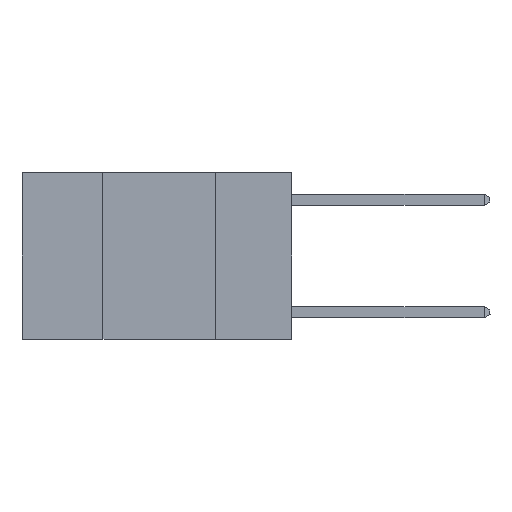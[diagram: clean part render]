
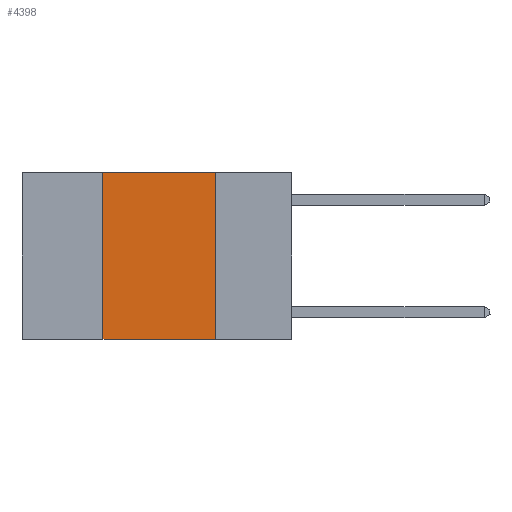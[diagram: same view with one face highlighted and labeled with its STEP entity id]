
A CAD part, left-side view. The second image highlights one B-rep face of the part: STEP entity #4398.
In plain terms, the highlighted planar face has unit normal (-1, 0, 0).
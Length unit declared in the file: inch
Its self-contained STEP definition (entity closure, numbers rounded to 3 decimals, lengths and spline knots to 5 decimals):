
#544 = CARTESIAN_POINT ( 'NONE',  ( 0., 0.17, 0. ) ) ;
#612 = CARTESIAN_POINT ( 'NONE',  ( 0., 0.17, -0.37 ) ) ;
#868 = EDGE_CURVE ( 'NONE', #10173, #6246, #11336, .T. ) ;
#2026 = VECTOR ( 'NONE', #4813, 39.37008 ) ;
#2029 = ORIENTED_EDGE ( 'NONE', *, *, #3747, .F. ) ;
#2306 = VERTEX_POINT ( 'NONE', #544 ) ;
#2623 = VECTOR ( 'NONE', #9434, 39.37008 ) ;
#3747 = EDGE_CURVE ( 'NONE', #2306, #5286, #10767, .T. ) ;
#3862 = EDGE_CURVE ( 'NONE', #10173, #5286, #4146, .T. ) ;
#3988 = ORIENTED_EDGE ( 'NONE', *, *, #3862, .T. ) ;
#4146 = LINE ( 'NONE', #8039, #8709 ) ;
#4253 = CARTESIAN_POINT ( 'NONE',  ( 0., 0.42, 0. ) ) ;
#4398 = ADVANCED_FACE ( 'NONE', ( #5860 ), #8008, .F. ) ;
#4813 = DIRECTION ( 'NONE',  ( 0., 0., 1. ) ) ;
#5286 = VERTEX_POINT ( 'NONE', #612 ) ;
#5776 = EDGE_CURVE ( 'NONE', #6246, #2306, #7367, .T. ) ;
#5856 = VECTOR ( 'NONE', #11482, 39.37008 ) ;
#5860 = FACE_OUTER_BOUND ( 'NONE', #10255, .T. ) ;
#6067 = CARTESIAN_POINT ( 'NONE',  ( 0., 0.42, -0.37 ) ) ;
#6246 = VERTEX_POINT ( 'NONE', #7239 ) ;
#7239 = CARTESIAN_POINT ( 'NONE',  ( 0., 0.42, 0. ) ) ;
#7367 = LINE ( 'NONE', #7677, #2623 ) ;
#7477 = AXIS2_PLACEMENT_3D ( 'NONE', #7942, #7882, #7865 ) ;
#7677 = CARTESIAN_POINT ( 'NONE',  ( 0., 0.6, 0. ) ) ;
#7780 = ORIENTED_EDGE ( 'NONE', *, *, #868, .F. ) ;
#7865 = DIRECTION ( 'NONE',  ( 0., 0., -1. ) ) ;
#7882 = DIRECTION ( 'NONE',  ( 1., 0., 0. ) ) ;
#7942 = CARTESIAN_POINT ( 'NONE',  ( 0., 0.6, 0. ) ) ;
#8008 = PLANE ( 'NONE',  #7477 ) ;
#8039 = CARTESIAN_POINT ( 'NONE',  ( 0., 0.6, -0.37 ) ) ;
#8063 = DIRECTION ( 'NONE',  ( 0., -1., 0. ) ) ;
#8709 = VECTOR ( 'NONE', #8063, 39.37008 ) ;
#9434 = DIRECTION ( 'NONE',  ( 0., -1., 0. ) ) ;
#9814 = ORIENTED_EDGE ( 'NONE', *, *, #5776, .F. ) ;
#10173 = VERTEX_POINT ( 'NONE', #6067 ) ;
#10255 = EDGE_LOOP ( 'NONE', ( #2029, #9814, #7780, #3988 ) ) ;
#10767 = LINE ( 'NONE', #11736, #5856 ) ;
#11336 = LINE ( 'NONE', #4253, #2026 ) ;
#11482 = DIRECTION ( 'NONE',  ( 0., 0., -1. ) ) ;
#11736 = CARTESIAN_POINT ( 'NONE',  ( 0., 0.17, 0. ) ) ;
